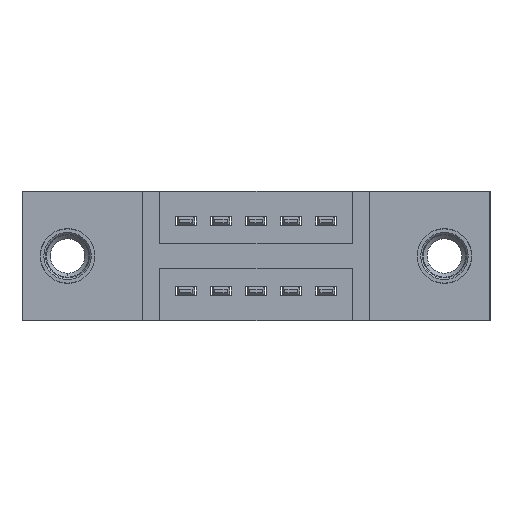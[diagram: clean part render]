
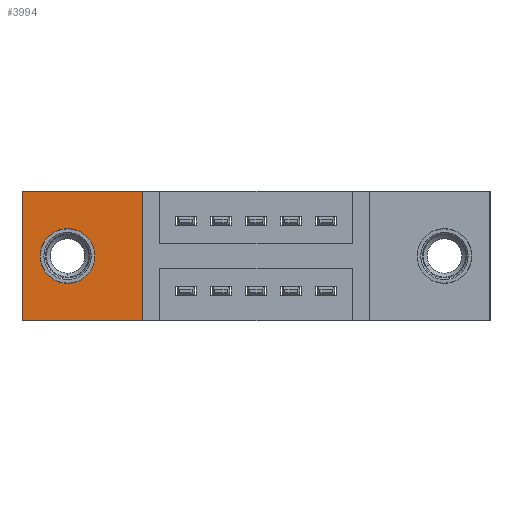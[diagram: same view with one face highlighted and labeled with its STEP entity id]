
A CAD part, front view. The second image highlights one B-rep face of the part: STEP entity #3994.
In plain terms, the highlighted planar face has unit normal (0, -1, 0).
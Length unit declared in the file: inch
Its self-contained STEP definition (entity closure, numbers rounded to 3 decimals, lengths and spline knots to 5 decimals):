
#444 = VECTOR ( 'NONE', #9364, 39.37008 ) ;
#834 = VECTOR ( 'NONE', #2988, 39.37008 ) ;
#840 = CARTESIAN_POINT ( 'NONE',  ( 0., 0.17, -0.37 ) ) ;
#858 = EDGE_CURVE ( 'NONE', #6346, #1787, #7395, .T. ) ;
#1146 = EDGE_CURVE ( 'NONE', #2680, #6346, #7868, .T. ) ;
#1588 = CARTESIAN_POINT ( 'NONE',  ( 0., 0.17, -0.37 ) ) ;
#1623 = EDGE_CURVE ( 'NONE', #2281, #1903, #5896, .T. ) ;
#1736 = CIRCLE ( 'NONE', #3438, 0.078 ) ;
#1787 = VERTEX_POINT ( 'NONE', #6483 ) ;
#1903 = VERTEX_POINT ( 'NONE', #5869 ) ;
#2136 = LINE ( 'NONE', #7040, #444 ) ;
#2281 = VERTEX_POINT ( 'NONE', #9841 ) ;
#2318 = PLANE ( 'NONE',  #5342 ) ;
#2342 = CARTESIAN_POINT ( 'NONE',  ( 0., 0.17, 0. ) ) ;
#2353 = DIRECTION ( 'NONE',  ( 0., -1., 0. ) ) ;
#2391 = CARTESIAN_POINT ( 'NONE',  ( 0.3425, 0.17, 0. ) ) ;
#2470 = DIRECTION ( 'NONE',  ( 0., -1., 0. ) ) ;
#2680 = VERTEX_POINT ( 'NONE', #3310 ) ;
#2882 = CARTESIAN_POINT ( 'NONE',  ( 0., 0.17, 0. ) ) ;
#2988 = DIRECTION ( 'NONE',  ( 0., 0., 1. ) ) ;
#3122 = DIRECTION ( 'NONE',  ( -1., 0., 0. ) ) ;
#3128 = CARTESIAN_POINT ( 'NONE',  ( 0.13, 0.17, -0.185 ) ) ;
#3147 = EDGE_LOOP ( 'NONE', ( #5265, #4223 ) ) ;
#3222 = DIRECTION ( 'NONE',  ( 0., 0., -1. ) ) ;
#3310 = CARTESIAN_POINT ( 'NONE',  ( 0.3425, 0.17, -0.37 ) ) ;
#3313 = EDGE_CURVE ( 'NONE', #5891, #2680, #2136, .T. ) ;
#3438 = AXIS2_PLACEMENT_3D ( 'NONE', #7912, #9418, #3222 ) ;
#3738 = ORIENTED_EDGE ( 'NONE', *, *, #3313, .T. ) ;
#3883 = EDGE_CURVE ( 'NONE', #1787, #5891, #9550, .T. ) ;
#3994 = ADVANCED_FACE ( 'NONE', ( #8569, #6729 ), #2318, .T. ) ;
#4223 = ORIENTED_EDGE ( 'NONE', *, *, #9676, .F. ) ;
#4513 = EDGE_LOOP ( 'NONE', ( #5494, #3738, #4900, #4822 ) ) ;
#4585 = VECTOR ( 'NONE', #3122, 39.37008 ) ;
#4822 = ORIENTED_EDGE ( 'NONE', *, *, #858, .T. ) ;
#4900 = ORIENTED_EDGE ( 'NONE', *, *, #1146, .T. ) ;
#5265 = ORIENTED_EDGE ( 'NONE', *, *, #1623, .F. ) ;
#5342 = AXIS2_PLACEMENT_3D ( 'NONE', #840, #2353, #5495 ) ;
#5494 = ORIENTED_EDGE ( 'NONE', *, *, #3883, .T. ) ;
#5495 = DIRECTION ( 'NONE',  ( 0., 0., -1. ) ) ;
#5526 = DIRECTION ( 'NONE',  ( 0., 0., -1. ) ) ;
#5869 = CARTESIAN_POINT ( 'NONE',  ( 0.13, 0.17, -0.263 ) ) ;
#5891 = VERTEX_POINT ( 'NONE', #1588 ) ;
#5896 = CIRCLE ( 'NONE', #8541, 0.078 ) ;
#6346 = VERTEX_POINT ( 'NONE', #2391 ) ;
#6483 = CARTESIAN_POINT ( 'NONE',  ( 0., 0.17, 0. ) ) ;
#6490 = VECTOR ( 'NONE', #8338, 39.37008 ) ;
#6729 = FACE_OUTER_BOUND ( 'NONE', #4513, .T. ) ;
#6866 = CARTESIAN_POINT ( 'NONE',  ( 0.3425, 0.17, 0. ) ) ;
#7040 = CARTESIAN_POINT ( 'NONE',  ( 0., 0.17, -0.37 ) ) ;
#7395 = LINE ( 'NONE', #2342, #4585 ) ;
#7868 = LINE ( 'NONE', #6866, #834 ) ;
#7912 = CARTESIAN_POINT ( 'NONE',  ( 0.13, 0.17, -0.185 ) ) ;
#8338 = DIRECTION ( 'NONE',  ( 0., 0., -1. ) ) ;
#8541 = AXIS2_PLACEMENT_3D ( 'NONE', #3128, #2470, #5526 ) ;
#8569 = FACE_BOUND ( 'NONE', #3147, .T. ) ;
#9364 = DIRECTION ( 'NONE',  ( 1., 0., 0. ) ) ;
#9418 = DIRECTION ( 'NONE',  ( 0., -1., 0. ) ) ;
#9550 = LINE ( 'NONE', #2882, #6490 ) ;
#9676 = EDGE_CURVE ( 'NONE', #1903, #2281, #1736, .T. ) ;
#9841 = CARTESIAN_POINT ( 'NONE',  ( 0.13, 0.17, -0.107 ) ) ;
